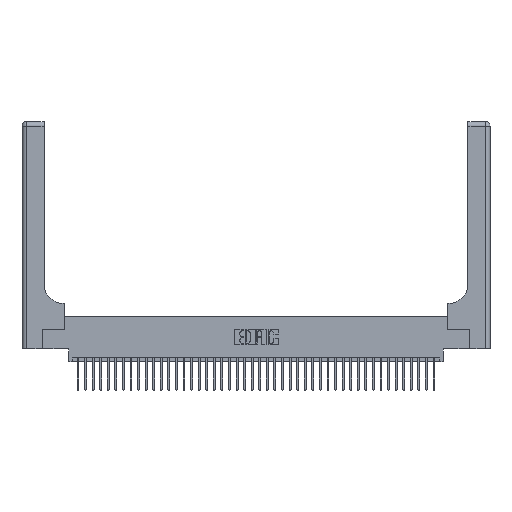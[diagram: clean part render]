
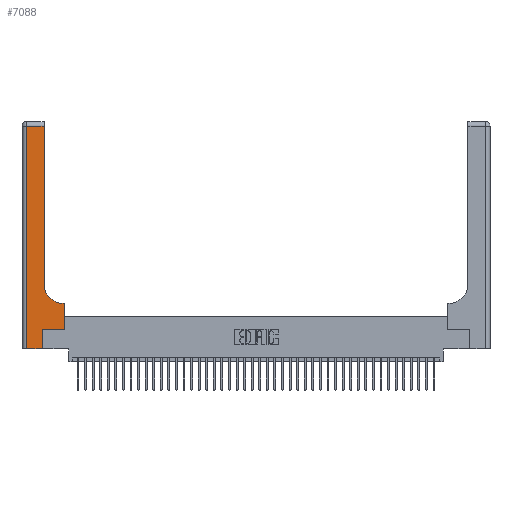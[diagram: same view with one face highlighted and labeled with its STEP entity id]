
A CAD part, top view. The second image highlights one B-rep face of the part: STEP entity #7088.
In plain terms, the highlighted planar face has unit normal (0, 0, 1).
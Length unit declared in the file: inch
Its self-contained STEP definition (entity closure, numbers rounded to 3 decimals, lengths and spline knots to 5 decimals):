
#517 = EDGE_CURVE ( 'NONE', #24289, #34158, #26650, .T. ) ;
#763 = PLANE ( 'NONE',  #5312 ) ;
#906 = EDGE_CURVE ( 'NONE', #12347, #12862, #17543, .T. ) ;
#1715 = VERTEX_POINT ( 'NONE', #3260 ) ;
#1918 = ORIENTED_EDGE ( 'NONE', *, *, #31371, .T. ) ;
#2306 = AXIS2_PLACEMENT_3D ( 'NONE', #17908, #5092, #4961 ) ;
#3260 = CARTESIAN_POINT ( 'NONE',  ( 0.06, 0., 0.37 ) ) ;
#3766 = ORIENTED_EDGE ( 'NONE', *, *, #906, .T. ) ;
#3911 = DIRECTION ( 'NONE',  ( 1., 0., 0. ) ) ;
#4151 = ORIENTED_EDGE ( 'NONE', *, *, #9504, .T. ) ;
#4441 = EDGE_CURVE ( 'NONE', #34158, #12347, #39127, .T. ) ;
#4558 = LINE ( 'NONE', #27956, #5085 ) ;
#4918 = LINE ( 'NONE', #7428, #33408 ) ;
#4961 = DIRECTION ( 'NONE',  ( 1., 0., 0. ) ) ;
#5085 = VECTOR ( 'NONE', #21634, 39.37008 ) ;
#5092 = DIRECTION ( 'NONE',  ( 0., 0., -1. ) ) ;
#5200 = CARTESIAN_POINT ( 'NONE',  ( 0.269, 0., 0.37 ) ) ;
#5213 = LINE ( 'NONE', #30235, #7248 ) ;
#5312 = AXIS2_PLACEMENT_3D ( 'NONE', #23577, #7349, #36816 ) ;
#5395 = CARTESIAN_POINT ( 'NONE',  ( 0.2915, 0.6, 0.37 ) ) ;
#6305 = VERTEX_POINT ( 'NONE', #5200 ) ;
#7088 = ADVANCED_FACE ( 'NONE', ( #22445 ), #763, .F. ) ;
#7248 = VECTOR ( 'NONE', #3911, 39.37008 ) ;
#7322 = CARTESIAN_POINT ( 'NONE',  ( 0.2915, 0.85, 0.37 ) ) ;
#7349 = DIRECTION ( 'NONE',  ( 0., 0., -1. ) ) ;
#7428 = CARTESIAN_POINT ( 'NONE',  ( 0., 2.94, 0.37 ) ) ;
#7938 = CARTESIAN_POINT ( 'NONE',  ( 0.269, 0.25, 0.37 ) ) ;
#8712 = ORIENTED_EDGE ( 'NONE', *, *, #4441, .T. ) ;
#8939 = ORIENTED_EDGE ( 'NONE', *, *, #40986, .T. ) ;
#9504 = EDGE_CURVE ( 'NONE', #35152, #15988, #4918, .T. ) ;
#9654 = DIRECTION ( 'NONE',  ( 0., 1., 0. ) ) ;
#10462 = VERTEX_POINT ( 'NONE', #7322 ) ;
#12347 = VERTEX_POINT ( 'NONE', #37424 ) ;
#12859 = DIRECTION ( 'NONE',  ( 1., 0., 0. ) ) ;
#12862 = VERTEX_POINT ( 'NONE', #24575 ) ;
#12963 = VECTOR ( 'NONE', #9654, 39.37008 ) ;
#13438 = ORIENTED_EDGE ( 'NONE', *, *, #517, .T. ) ;
#15196 = ORIENTED_EDGE ( 'NONE', *, *, #40548, .T. ) ;
#15749 = EDGE_CURVE ( 'NONE', #6305, #24289, #4558, .T. ) ;
#15988 = VERTEX_POINT ( 'NONE', #39409 ) ;
#16095 = VECTOR ( 'NONE', #41573, 39.37008 ) ;
#16115 = DIRECTION ( 'NONE',  ( 0., 1., 0. ) ) ;
#16543 = CIRCLE ( 'NONE', #2306, 0.25 ) ;
#17543 = LINE ( 'NONE', #5395, #32777 ) ;
#17779 = ORIENTED_EDGE ( 'NONE', *, *, #15749, .T. ) ;
#17908 = CARTESIAN_POINT ( 'NONE',  ( 0.5415, 0.85, 0.37 ) ) ;
#19533 = ORIENTED_EDGE ( 'NONE', *, *, #41662, .T. ) ;
#21634 = DIRECTION ( 'NONE',  ( 0., 1., 0. ) ) ;
#22445 = FACE_OUTER_BOUND ( 'NONE', #24131, .T. ) ;
#23577 = CARTESIAN_POINT ( 'NONE',  ( 0., 3., 0.37 ) ) ;
#23669 = LINE ( 'NONE', #29806, #12963 ) ;
#24083 = DIRECTION ( 'NONE',  ( -1., 0., 0. ) ) ;
#24131 = EDGE_LOOP ( 'NONE', ( #19533, #4151, #15196, #1918, #17779, #13438, #8712, #3766, #8939 ) ) ;
#24289 = VERTEX_POINT ( 'NONE', #7938 ) ;
#24575 = CARTESIAN_POINT ( 'NONE',  ( 0.5415, 0.6, 0.37 ) ) ;
#24805 = LINE ( 'NONE', #25217, #16095 ) ;
#25217 = CARTESIAN_POINT ( 'NONE',  ( 0.06, 3., 0.37 ) ) ;
#25557 = CARTESIAN_POINT ( 'NONE',  ( 0.2915, 2.94, 0.37 ) ) ;
#26650 = LINE ( 'NONE', #28008, #27697 ) ;
#27697 = VECTOR ( 'NONE', #12859, 39.37008 ) ;
#27942 = DIRECTION ( 'NONE',  ( -1., 0., 0. ) ) ;
#27956 = CARTESIAN_POINT ( 'NONE',  ( 0.269, 0., 0.37 ) ) ;
#28008 = CARTESIAN_POINT ( 'NONE',  ( 0.269, 0.25, 0.37 ) ) ;
#29806 = CARTESIAN_POINT ( 'NONE',  ( 0.2915, 3., 0.37 ) ) ;
#30235 = CARTESIAN_POINT ( 'NONE',  ( 0., 0., 0.37 ) ) ;
#31371 = EDGE_CURVE ( 'NONE', #1715, #6305, #5213, .T. ) ;
#31963 = VECTOR ( 'NONE', #16115, 39.37008 ) ;
#32777 = VECTOR ( 'NONE', #27942, 39.37008 ) ;
#33408 = VECTOR ( 'NONE', #24083, 39.37008 ) ;
#34158 = VERTEX_POINT ( 'NONE', #39071 ) ;
#35152 = VERTEX_POINT ( 'NONE', #25557 ) ;
#36816 = DIRECTION ( 'NONE',  ( -1., 0., 0. ) ) ;
#37424 = CARTESIAN_POINT ( 'NONE',  ( 0.5585, 0.6, 0.37 ) ) ;
#38778 = CARTESIAN_POINT ( 'NONE',  ( 0.5585, 0.25, 0.37 ) ) ;
#39071 = CARTESIAN_POINT ( 'NONE',  ( 0.5585, 0.25, 0.37 ) ) ;
#39127 = LINE ( 'NONE', #38778, #31963 ) ;
#39409 = CARTESIAN_POINT ( 'NONE',  ( 0.06, 2.94, 0.37 ) ) ;
#40548 = EDGE_CURVE ( 'NONE', #15988, #1715, #24805, .T. ) ;
#40986 = EDGE_CURVE ( 'NONE', #12862, #10462, #16543, .T. ) ;
#41573 = DIRECTION ( 'NONE',  ( 0., -1., 0. ) ) ;
#41662 = EDGE_CURVE ( 'NONE', #10462, #35152, #23669, .T. ) ;
